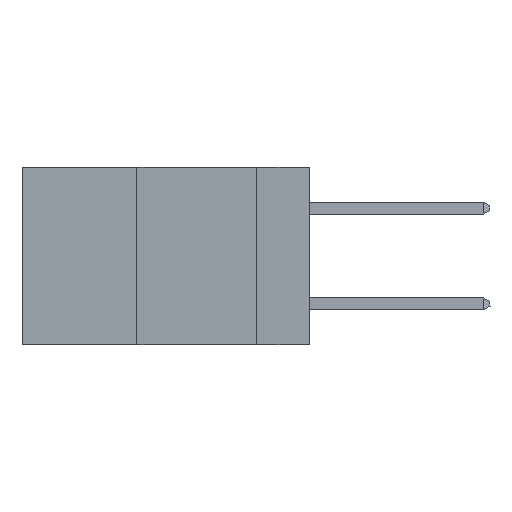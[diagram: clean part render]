
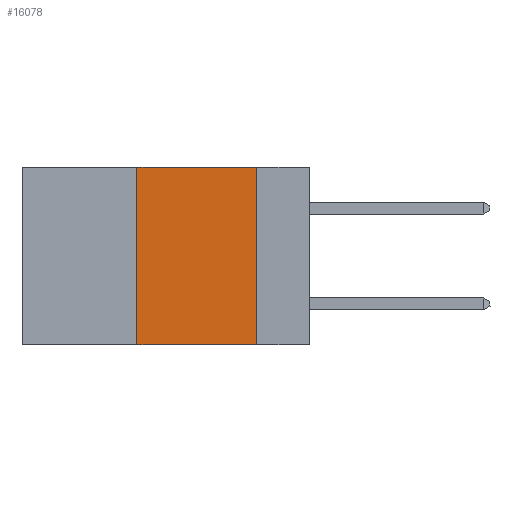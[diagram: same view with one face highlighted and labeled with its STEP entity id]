
A CAD part, left-side view. The second image highlights one B-rep face of the part: STEP entity #16078.
In plain terms, the highlighted planar face has unit normal (-1, 0, 0).
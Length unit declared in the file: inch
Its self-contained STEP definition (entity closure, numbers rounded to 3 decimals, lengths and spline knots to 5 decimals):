
#1188 = LINE ( 'NONE', #6638, #14716 ) ;
#1412 = VERTEX_POINT ( 'NONE', #11921 ) ;
#2007 = EDGE_LOOP ( 'NONE', ( #5370, #5716, #5935, #5986 ) ) ;
#2638 = AXIS2_PLACEMENT_3D ( 'NONE', #20624, #10229, #22324 ) ;
#2700 = DIRECTION ( 'NONE',  ( 0., -1., 0. ) ) ;
#5370 = ORIENTED_EDGE ( 'NONE', *, *, #7520, .F. ) ;
#5716 = ORIENTED_EDGE ( 'NONE', *, *, #19603, .F. ) ;
#5769 = VERTEX_POINT ( 'NONE', #14665 ) ;
#5935 = ORIENTED_EDGE ( 'NONE', *, *, #11429, .F. ) ;
#5986 = ORIENTED_EDGE ( 'NONE', *, *, #22116, .T. ) ;
#6638 = CARTESIAN_POINT ( 'NONE',  ( 0., 0.36, 0. ) ) ;
#6717 = PLANE ( 'NONE',  #2638 ) ;
#7520 = EDGE_CURVE ( 'NONE', #5769, #8630, #13184, .T. ) ;
#8309 = LINE ( 'NONE', #21908, #16536 ) ;
#8372 = DIRECTION ( 'NONE',  ( 0., 0., 1. ) ) ;
#8491 = VECTOR ( 'NONE', #2700, 39.37008 ) ;
#8630 = VERTEX_POINT ( 'NONE', #9200 ) ;
#8679 = FACE_OUTER_BOUND ( 'NONE', #2007, .T. ) ;
#9200 = CARTESIAN_POINT ( 'NONE',  ( 0., 0.11, -0.37 ) ) ;
#9798 = DIRECTION ( 'NONE',  ( 0., -1., 0. ) ) ;
#10229 = DIRECTION ( 'NONE',  ( 1., 0., 0. ) ) ;
#11429 = EDGE_CURVE ( 'NONE', #1412, #16401, #1188, .T. ) ;
#11921 = CARTESIAN_POINT ( 'NONE',  ( 0., 0.36, -0.37 ) ) ;
#13184 = LINE ( 'NONE', #19726, #21245 ) ;
#13269 = CARTESIAN_POINT ( 'NONE',  ( 0., 0.6, -0.37 ) ) ;
#14665 = CARTESIAN_POINT ( 'NONE',  ( 0., 0.11, 0. ) ) ;
#14716 = VECTOR ( 'NONE', #8372, 39.37008 ) ;
#16078 = ADVANCED_FACE ( 'NONE', ( #8679 ), #6717, .F. ) ;
#16401 = VERTEX_POINT ( 'NONE', #21517 ) ;
#16536 = VECTOR ( 'NONE', #9798, 39.37008 ) ;
#17800 = LINE ( 'NONE', #13269, #8491 ) ;
#19603 = EDGE_CURVE ( 'NONE', #16401, #5769, #8309, .T. ) ;
#19726 = CARTESIAN_POINT ( 'NONE',  ( 0., 0.11, 0. ) ) ;
#20624 = CARTESIAN_POINT ( 'NONE',  ( 0., 0.6, 0. ) ) ;
#21245 = VECTOR ( 'NONE', #21447, 39.37008 ) ;
#21447 = DIRECTION ( 'NONE',  ( 0., 0., -1. ) ) ;
#21517 = CARTESIAN_POINT ( 'NONE',  ( 0., 0.36, 0. ) ) ;
#21908 = CARTESIAN_POINT ( 'NONE',  ( 0., 0.6, 0. ) ) ;
#22116 = EDGE_CURVE ( 'NONE', #1412, #8630, #17800, .T. ) ;
#22324 = DIRECTION ( 'NONE',  ( 0., 0., -1. ) ) ;
